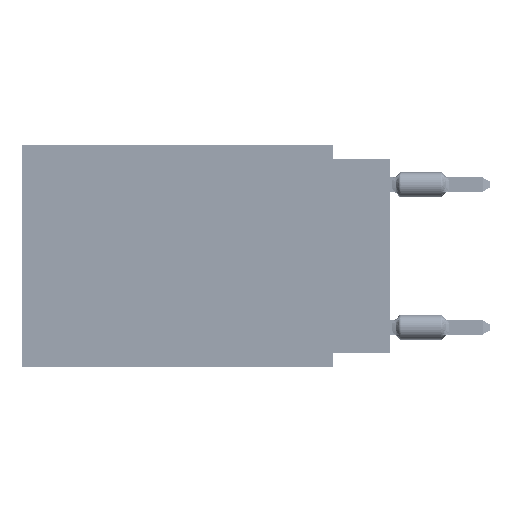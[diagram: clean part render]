
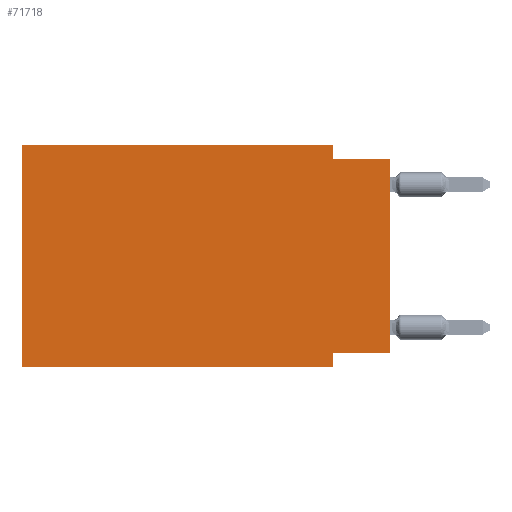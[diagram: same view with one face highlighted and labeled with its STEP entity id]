
A CAD part, left-side view. The second image highlights one B-rep face of the part: STEP entity #71718.
In plain terms, the highlighted planar face has unit normal (-1, 0, 0).
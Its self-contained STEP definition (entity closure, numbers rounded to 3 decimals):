
#421 = VERTEX_POINT ( 'NONE', #82983 ) ;
#3760 = CARTESIAN_POINT ( 'NONE',  ( 0., 16.383, -9.906 ) ) ;
#3866 = ORIENTED_EDGE ( 'NONE', *, *, #75128, .F. ) ;
#4006 = CARTESIAN_POINT ( 'NONE',  ( 0., 0., -0.635 ) ) ;
#4247 = CARTESIAN_POINT ( 'NONE',  ( 0., 16.383, 0. ) ) ;
#7300 = EDGE_CURVE ( 'NONE', #52521, #52088, #22142, .T. ) ;
#7822 = CARTESIAN_POINT ( 'NONE',  ( 0., 2.54, 0. ) ) ;
#11538 = DIRECTION ( 'NONE',  ( 0., 0., 1. ) ) ;
#14237 = LINE ( 'NONE', #7822, #76407 ) ;
#17111 = EDGE_CURVE ( 'NONE', #48747, #421, #68846, .T. ) ;
#17130 = EDGE_CURVE ( 'NONE', #51012, #44804, #56441, .T. ) ;
#19017 = VECTOR ( 'NONE', #66935, 1000. ) ;
#21997 = PLANE ( 'NONE',  #23418 ) ;
#22142 = LINE ( 'NONE', #41838, #73563 ) ;
#23418 = AXIS2_PLACEMENT_3D ( 'NONE', #36117, #48117, #42516 ) ;
#27252 = ORIENTED_EDGE ( 'NONE', *, *, #80047, .F. ) ;
#29256 = VECTOR ( 'NONE', #60465, 1000. ) ;
#30247 = DIRECTION ( 'NONE',  ( 0., -1., 0. ) ) ;
#32179 = VECTOR ( 'NONE', #61598, 1000. ) ;
#32547 = CARTESIAN_POINT ( 'NONE',  ( 0., 16.383, -9.906 ) ) ;
#32713 = CARTESIAN_POINT ( 'NONE',  ( 0., 2.54, -9.271 ) ) ;
#36117 = CARTESIAN_POINT ( 'NONE',  ( 0., 16.383, 0. ) ) ;
#36542 = EDGE_CURVE ( 'NONE', #56883, #44804, #41618, .T. ) ;
#40345 = CARTESIAN_POINT ( 'NONE',  ( 0., 0., 0. ) ) ;
#40831 = CARTESIAN_POINT ( 'NONE',  ( 0., 2.54, -9.906 ) ) ;
#41618 = LINE ( 'NONE', #40345, #29256 ) ;
#41838 = CARTESIAN_POINT ( 'NONE',  ( 0., 16.383, 0. ) ) ;
#41905 = CARTESIAN_POINT ( 'NONE',  ( 0., 0., -0.635 ) ) ;
#42516 = DIRECTION ( 'NONE',  ( 0., 0., -1. ) ) ;
#44568 = VECTOR ( 'NONE', #11538, 1000. ) ;
#44804 = VERTEX_POINT ( 'NONE', #4006 ) ;
#47183 = EDGE_LOOP ( 'NONE', ( #52397, #58233, #27252, #64365, #66372, #65009, #63915, #3866 ) ) ;
#47251 = LINE ( 'NONE', #40831, #19017 ) ;
#47623 = DIRECTION ( 'NONE',  ( 0., 0., -1. ) ) ;
#48117 = DIRECTION ( 'NONE',  ( 1., 0., 0. ) ) ;
#48747 = VERTEX_POINT ( 'NONE', #32547 ) ;
#49103 = LINE ( 'NONE', #81227, #60838 ) ;
#51012 = VERTEX_POINT ( 'NONE', #74897 ) ;
#52088 = VERTEX_POINT ( 'NONE', #53233 ) ;
#52397 = ORIENTED_EDGE ( 'NONE', *, *, #36542, .T. ) ;
#52521 = VERTEX_POINT ( 'NONE', #72829 ) ;
#53233 = CARTESIAN_POINT ( 'NONE',  ( 0., 2.54, 0. ) ) ;
#56441 = LINE ( 'NONE', #41905, #78663 ) ;
#56883 = VERTEX_POINT ( 'NONE', #76274 ) ;
#58233 = ORIENTED_EDGE ( 'NONE', *, *, #17130, .F. ) ;
#60465 = DIRECTION ( 'NONE',  ( 0., 0., 1. ) ) ;
#60838 = VECTOR ( 'NONE', #75203, 1000. ) ;
#61598 = DIRECTION ( 'NONE',  ( 0., -1., 0. ) ) ;
#63513 = VERTEX_POINT ( 'NONE', #32713 ) ;
#63695 = EDGE_CURVE ( 'NONE', #63513, #421, #47251, .T. ) ;
#63915 = ORIENTED_EDGE ( 'NONE', *, *, #63695, .F. ) ;
#64365 = ORIENTED_EDGE ( 'NONE', *, *, #7300, .F. ) ;
#65009 = ORIENTED_EDGE ( 'NONE', *, *, #17111, .T. ) ;
#66372 = ORIENTED_EDGE ( 'NONE', *, *, #76450, .F. ) ;
#66935 = DIRECTION ( 'NONE',  ( 0., 0., -1. ) ) ;
#68020 = DIRECTION ( 'NONE',  ( 0., -1., 0. ) ) ;
#68846 = LINE ( 'NONE', #3760, #32179 ) ;
#69751 = LINE ( 'NONE', #4247, #44568 ) ;
#71718 = ADVANCED_FACE ( 'NONE', ( #74644 ), #21997, .F. ) ;
#72829 = CARTESIAN_POINT ( 'NONE',  ( 0., 16.383, 0. ) ) ;
#73563 = VECTOR ( 'NONE', #30247, 1000. ) ;
#74644 = FACE_OUTER_BOUND ( 'NONE', #47183, .T. ) ;
#74897 = CARTESIAN_POINT ( 'NONE',  ( 0., 2.54, -0.635 ) ) ;
#75128 = EDGE_CURVE ( 'NONE', #56883, #63513, #49103, .T. ) ;
#75203 = DIRECTION ( 'NONE',  ( 0., 1., 0. ) ) ;
#76274 = CARTESIAN_POINT ( 'NONE',  ( 0., 0., -9.271 ) ) ;
#76407 = VECTOR ( 'NONE', #47623, 1000. ) ;
#76450 = EDGE_CURVE ( 'NONE', #48747, #52521, #69751, .T. ) ;
#78663 = VECTOR ( 'NONE', #68020, 1000. ) ;
#80047 = EDGE_CURVE ( 'NONE', #52088, #51012, #14237, .T. ) ;
#81227 = CARTESIAN_POINT ( 'NONE',  ( 0., 0., -9.271 ) ) ;
#82983 = CARTESIAN_POINT ( 'NONE',  ( 0., 2.54, -9.906 ) ) ;
